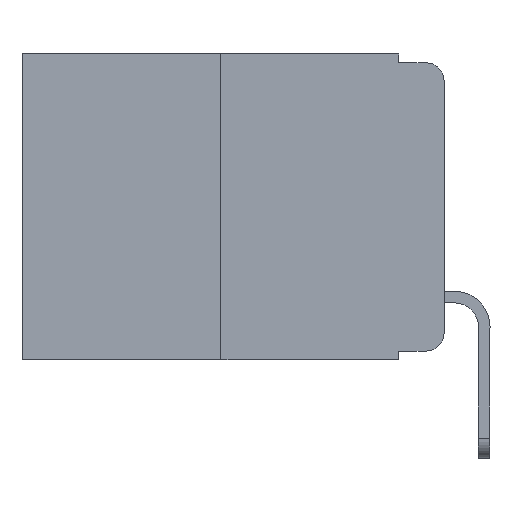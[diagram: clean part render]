
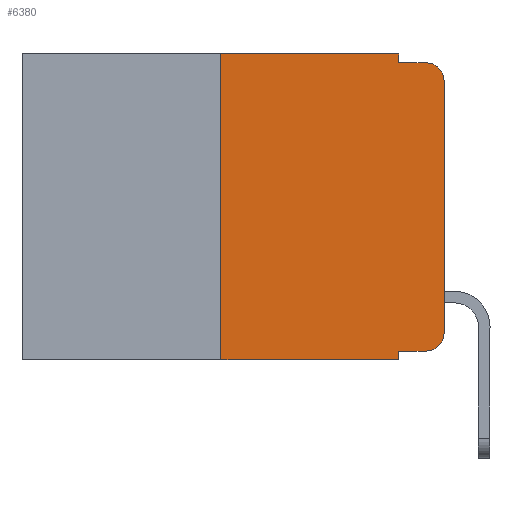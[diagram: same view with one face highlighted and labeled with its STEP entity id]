
A CAD part, left-side view. The second image highlights one B-rep face of the part: STEP entity #6380.
In plain terms, the highlighted planar face has unit normal (-1, 0, 0).
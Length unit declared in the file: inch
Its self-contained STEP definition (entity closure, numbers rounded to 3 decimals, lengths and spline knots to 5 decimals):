
#290 = VERTEX_POINT ( 'NONE', #8452 ) ;
#631 = VERTEX_POINT ( 'NONE', #4201 ) ;
#1217 = EDGE_CURVE ( 'NONE', #631, #1379, #17402, .T. ) ;
#1255 = AXIS2_PLACEMENT_3D ( 'NONE', #22575, #8706, #20994 ) ;
#1333 = ORIENTED_EDGE ( 'NONE', *, *, #8759, .F. ) ;
#1379 = VERTEX_POINT ( 'NONE', #17064 ) ;
#1385 = CARTESIAN_POINT ( 'NONE',  ( 0., 0., -0.313 ) ) ;
#1475 = DIRECTION ( 'NONE',  ( -1., 0., 0. ) ) ;
#1786 = CARTESIAN_POINT ( 'NONE',  ( 0., 0.051, 0. ) ) ;
#1961 = CARTESIAN_POINT ( 'NONE',  ( 0., 0.473, -0.343 ) ) ;
#2126 = LINE ( 'NONE', #20541, #12163 ) ;
#2788 = ORIENTED_EDGE ( 'NONE', *, *, #1217, .F. ) ;
#2902 = EDGE_LOOP ( 'NONE', ( #20211, #20729, #1333, #16721, #2788, #13188, #22262, #18141, #22529, #15622 ) ) ;
#3694 = VERTEX_POINT ( 'NONE', #1385 ) ;
#4201 = CARTESIAN_POINT ( 'NONE',  ( 0., 0.25, 0. ) ) ;
#4861 = LINE ( 'NONE', #5833, #14297 ) ;
#5504 = CIRCLE ( 'NONE', #11483, 0.02 ) ;
#5833 = CARTESIAN_POINT ( 'NONE',  ( 0., 0.051, -0.01 ) ) ;
#6380 = ADVANCED_FACE ( 'NONE', ( #7826 ), #10579, .F. ) ;
#6462 = CARTESIAN_POINT ( 'NONE',  ( 0., 0., -0.03 ) ) ;
#6956 = DIRECTION ( 'NONE',  ( 0., -1., 0. ) ) ;
#7559 = EDGE_CURVE ( 'NONE', #19487, #22778, #12412, .T. ) ;
#7745 = VECTOR ( 'NONE', #17105, 39.37008 ) ;
#7759 = CARTESIAN_POINT ( 'NONE',  ( 0., 0.02, -0.01 ) ) ;
#7826 = FACE_OUTER_BOUND ( 'NONE', #2902, .T. ) ;
#7890 = DIRECTION ( 'NONE',  ( 0., -1., 0. ) ) ;
#8295 = VERTEX_POINT ( 'NONE', #7759 ) ;
#8348 = LINE ( 'NONE', #1786, #13241 ) ;
#8411 = VECTOR ( 'NONE', #6956, 39.37008 ) ;
#8452 = CARTESIAN_POINT ( 'NONE',  ( 0., 0.051, -0.333 ) ) ;
#8477 = DIRECTION ( 'NONE',  ( -1., 0., 0. ) ) ;
#8633 = VERTEX_POINT ( 'NONE', #23054 ) ;
#8706 = DIRECTION ( 'NONE',  ( 1., 0., 0. ) ) ;
#8727 = EDGE_CURVE ( 'NONE', #3694, #22993, #16527, .T. ) ;
#8750 = EDGE_CURVE ( 'NONE', #22993, #8295, #5504, .T. ) ;
#8759 = EDGE_CURVE ( 'NONE', #14555, #8295, #4861, .T. ) ;
#8787 = EDGE_CURVE ( 'NONE', #1379, #14555, #8348, .T. ) ;
#8789 = EDGE_CURVE ( 'NONE', #19487, #631, #21797, .T. ) ;
#8795 = EDGE_CURVE ( 'NONE', #290, #22778, #2126, .T. ) ;
#8824 = EDGE_CURVE ( 'NONE', #290, #8633, #20780, .T. ) ;
#8858 = EDGE_CURVE ( 'NONE', #8633, #3694, #10485, .T. ) ;
#9213 = CARTESIAN_POINT ( 'NONE',  ( 0., 0.051, -0.01 ) ) ;
#10020 = CARTESIAN_POINT ( 'NONE',  ( 0., 0.25, 0. ) ) ;
#10485 = CIRCLE ( 'NONE', #16104, 0.02 ) ;
#10579 = PLANE ( 'NONE',  #1255 ) ;
#11483 = AXIS2_PLACEMENT_3D ( 'NONE', #13356, #1475, #15064 ) ;
#11883 = VECTOR ( 'NONE', #12096, 39.37008 ) ;
#12096 = DIRECTION ( 'NONE',  ( 0., -1., 0. ) ) ;
#12163 = VECTOR ( 'NONE', #22176, 39.37008 ) ;
#12412 = LINE ( 'NONE', #1961, #11883 ) ;
#12570 = CARTESIAN_POINT ( 'NONE',  ( 0., 0.25, -0.343 ) ) ;
#13153 = CARTESIAN_POINT ( 'NONE',  ( 0., 0., 0. ) ) ;
#13188 = ORIENTED_EDGE ( 'NONE', *, *, #8789, .F. ) ;
#13223 = DIRECTION ( 'NONE',  ( 0., 0., 1. ) ) ;
#13241 = VECTOR ( 'NONE', #15289, 39.37008 ) ;
#13356 = CARTESIAN_POINT ( 'NONE',  ( 0., 0.02, -0.03 ) ) ;
#13675 = CARTESIAN_POINT ( 'NONE',  ( 0., 0.051, -0.343 ) ) ;
#14297 = VECTOR ( 'NONE', #7890, 39.37008 ) ;
#14555 = VERTEX_POINT ( 'NONE', #9213 ) ;
#15064 = DIRECTION ( 'NONE',  ( 0., 0., -1. ) ) ;
#15289 = DIRECTION ( 'NONE',  ( 0., 0., -1. ) ) ;
#15622 = ORIENTED_EDGE ( 'NONE', *, *, #8858, .T. ) ;
#15962 = VECTOR ( 'NONE', #13223, 39.37008 ) ;
#16104 = AXIS2_PLACEMENT_3D ( 'NONE', #19141, #8477, #20817 ) ;
#16527 = LINE ( 'NONE', #13153, #15962 ) ;
#16721 = ORIENTED_EDGE ( 'NONE', *, *, #8787, .F. ) ;
#17064 = CARTESIAN_POINT ( 'NONE',  ( 0., 0.051, 0. ) ) ;
#17105 = DIRECTION ( 'NONE',  ( 0., 0., 1. ) ) ;
#17258 = CARTESIAN_POINT ( 'NONE',  ( 0., 0.051, -0.333 ) ) ;
#17402 = LINE ( 'NONE', #17881, #8411 ) ;
#17881 = CARTESIAN_POINT ( 'NONE',  ( 0., 0.473, 0. ) ) ;
#18141 = ORIENTED_EDGE ( 'NONE', *, *, #8795, .F. ) ;
#19141 = CARTESIAN_POINT ( 'NONE',  ( 0., 0.02, -0.313 ) ) ;
#19487 = VERTEX_POINT ( 'NONE', #12570 ) ;
#20211 = ORIENTED_EDGE ( 'NONE', *, *, #8727, .T. ) ;
#20266 = VECTOR ( 'NONE', #20680, 39.37008 ) ;
#20541 = CARTESIAN_POINT ( 'NONE',  ( 0., 0.051, 0. ) ) ;
#20680 = DIRECTION ( 'NONE',  ( 0., -1., 0. ) ) ;
#20729 = ORIENTED_EDGE ( 'NONE', *, *, #8750, .T. ) ;
#20780 = LINE ( 'NONE', #17258, #20266 ) ;
#20817 = DIRECTION ( 'NONE',  ( 0., 0., -1. ) ) ;
#20994 = DIRECTION ( 'NONE',  ( 0., 0., -1. ) ) ;
#21797 = LINE ( 'NONE', #10020, #7745 ) ;
#22176 = DIRECTION ( 'NONE',  ( 0., 0., -1. ) ) ;
#22262 = ORIENTED_EDGE ( 'NONE', *, *, #7559, .T. ) ;
#22529 = ORIENTED_EDGE ( 'NONE', *, *, #8824, .T. ) ;
#22575 = CARTESIAN_POINT ( 'NONE',  ( 0., 0.473, 0. ) ) ;
#22778 = VERTEX_POINT ( 'NONE', #13675 ) ;
#22993 = VERTEX_POINT ( 'NONE', #6462 ) ;
#23054 = CARTESIAN_POINT ( 'NONE',  ( 0., 0.02, -0.333 ) ) ;
